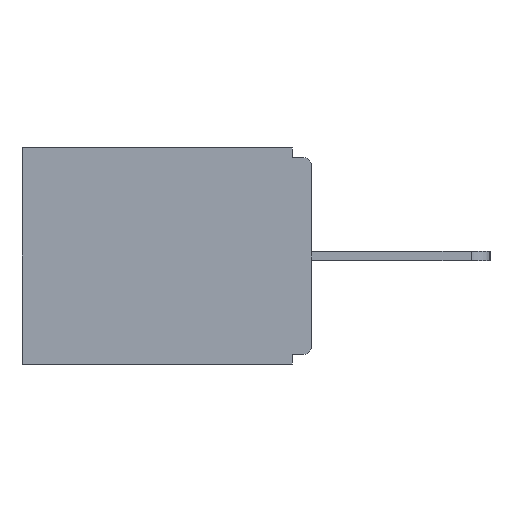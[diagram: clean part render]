
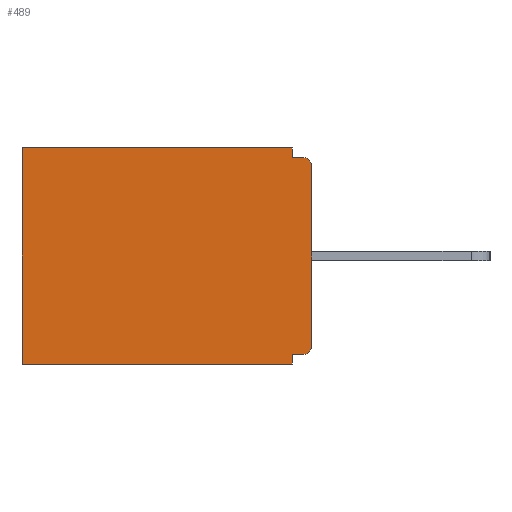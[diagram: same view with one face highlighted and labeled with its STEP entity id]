
A CAD part, left-side view. The second image highlights one B-rep face of the part: STEP entity #489.
In plain terms, the highlighted planar face has unit normal (-1, 0, 0).
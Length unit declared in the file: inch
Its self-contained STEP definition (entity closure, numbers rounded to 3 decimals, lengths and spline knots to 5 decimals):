
#12 = DIRECTION ( 'NONE',  ( 0., 0., -1. ) ) ;
#49 = ORIENTED_EDGE ( 'NONE', *, *, #7916, .T. ) ;
#286 = VECTOR ( 'NONE', #7599, 39.37008 ) ;
#290 = EDGE_CURVE ( 'NONE', #2444, #10010, #12416, .T. ) ;
#346 = CIRCLE ( 'NONE', #12971, 0.015 ) ;
#489 = ADVANCED_FACE ( 'NONE', ( #7421 ), #2189, .F. ) ;
#512 = LINE ( 'NONE', #12694, #10845 ) ;
#618 = DIRECTION ( 'NONE',  ( 0., -1., 0. ) ) ;
#804 = DIRECTION ( 'NONE',  ( 0., 0., -1. ) ) ;
#906 = ORIENTED_EDGE ( 'NONE', *, *, #11463, .F. ) ;
#972 = CARTESIAN_POINT ( 'NONE',  ( 0.298, 0.015, -0.313 ) ) ;
#1061 = CARTESIAN_POINT ( 'NONE',  ( 0.298, 0.015, -0.03 ) ) ;
#1147 = DIRECTION ( 'NONE',  ( -1., 0., 0. ) ) ;
#1415 = DIRECTION ( 'NONE',  ( 0., 1., 0. ) ) ;
#1557 = ORIENTED_EDGE ( 'NONE', *, *, #7293, .F. ) ;
#1739 = LINE ( 'NONE', #12682, #286 ) ;
#1891 = VERTEX_POINT ( 'NONE', #12522 ) ;
#1892 = DIRECTION ( 'NONE',  ( 0., 1., 0. ) ) ;
#1963 = ORIENTED_EDGE ( 'NONE', *, *, #5294, .T. ) ;
#2013 = LINE ( 'NONE', #12012, #6350 ) ;
#2139 = EDGE_LOOP ( 'NONE', ( #1963, #11850, #2563, #49, #9043, #9344, #906, #1557, #4140, #12208 ) ) ;
#2189 = PLANE ( 'NONE',  #11971 ) ;
#2194 = CARTESIAN_POINT ( 'NONE',  ( 0.298, 0.015, -0.015 ) ) ;
#2214 = CARTESIAN_POINT ( 'NONE',  ( 0.298, 0.031, -0.015 ) ) ;
#2283 = VECTOR ( 'NONE', #618, 39.37008 ) ;
#2444 = VERTEX_POINT ( 'NONE', #2214 ) ;
#2563 = ORIENTED_EDGE ( 'NONE', *, *, #6352, .F. ) ;
#2890 = CARTESIAN_POINT ( 'NONE',  ( 0.298, 0., -0.343 ) ) ;
#2955 = CARTESIAN_POINT ( 'NONE',  ( 0.298, 0., -0.03 ) ) ;
#2999 = CARTESIAN_POINT ( 'NONE',  ( 0.298, 0., 0. ) ) ;
#3053 = CARTESIAN_POINT ( 'NONE',  ( 0.298, 0.031, -0.328 ) ) ;
#3123 = LINE ( 'NONE', #12525, #12603 ) ;
#3130 = DIRECTION ( 'NONE',  ( 1., 0., 0. ) ) ;
#3139 = DIRECTION ( 'NONE',  ( 0., 0., -1. ) ) ;
#3141 = VECTOR ( 'NONE', #4086, 39.37008 ) ;
#3318 = EDGE_CURVE ( 'NONE', #7653, #8867, #8622, .T. ) ;
#4086 = DIRECTION ( 'NONE',  ( 0., 0., -1. ) ) ;
#4140 = ORIENTED_EDGE ( 'NONE', *, *, #5238, .T. ) ;
#4240 = CARTESIAN_POINT ( 'NONE',  ( 0.298, 0., 0. ) ) ;
#4428 = AXIS2_PLACEMENT_3D ( 'NONE', #972, #1147, #3139 ) ;
#5163 = DIRECTION ( 'NONE',  ( 0., 0., -1. ) ) ;
#5238 = EDGE_CURVE ( 'NONE', #5917, #8867, #8730, .T. ) ;
#5294 = EDGE_CURVE ( 'NONE', #7653, #10010, #346, .T. ) ;
#5343 = VERTEX_POINT ( 'NONE', #7398 ) ;
#5917 = VERTEX_POINT ( 'NONE', #8154 ) ;
#6086 = VERTEX_POINT ( 'NONE', #7644 ) ;
#6161 = EDGE_CURVE ( 'NONE', #1891, #5343, #11359, .T. ) ;
#6350 = VECTOR ( 'NONE', #804, 39.37008 ) ;
#6352 = EDGE_CURVE ( 'NONE', #6086, #2444, #3123, .T. ) ;
#6745 = CARTESIAN_POINT ( 'NONE',  ( 0.298, 0., -0.015 ) ) ;
#7293 = EDGE_CURVE ( 'NONE', #5917, #12135, #512, .T. ) ;
#7398 = CARTESIAN_POINT ( 'NONE',  ( 0.298, 0.46, -0.343 ) ) ;
#7421 = FACE_OUTER_BOUND ( 'NONE', #2139, .T. ) ;
#7599 = DIRECTION ( 'NONE',  ( 0., 0., -1. ) ) ;
#7644 = CARTESIAN_POINT ( 'NONE',  ( 0.298, 0.031, 0. ) ) ;
#7653 = VERTEX_POINT ( 'NONE', #2955 ) ;
#7916 = EDGE_CURVE ( 'NONE', #6086, #9658, #10833, .T. ) ;
#8071 = VECTOR ( 'NONE', #11411, 39.37008 ) ;
#8154 = CARTESIAN_POINT ( 'NONE',  ( 0.298, 0.015, -0.328 ) ) ;
#8622 = LINE ( 'NONE', #2999, #3141 ) ;
#8730 = CIRCLE ( 'NONE', #4428, 0.015 ) ;
#8867 = VERTEX_POINT ( 'NONE', #12286 ) ;
#9043 = ORIENTED_EDGE ( 'NONE', *, *, #9278, .T. ) ;
#9278 = EDGE_CURVE ( 'NONE', #9658, #5343, #1739, .T. ) ;
#9344 = ORIENTED_EDGE ( 'NONE', *, *, #6161, .F. ) ;
#9658 = VERTEX_POINT ( 'NONE', #11991 ) ;
#10010 = VERTEX_POINT ( 'NONE', #2194 ) ;
#10082 = VECTOR ( 'NONE', #1892, 39.37008 ) ;
#10272 = CARTESIAN_POINT ( 'NONE',  ( 0.298, 0., 0. ) ) ;
#10833 = LINE ( 'NONE', #4240, #8071 ) ;
#10845 = VECTOR ( 'NONE', #1415, 39.37008 ) ;
#11352 = DIRECTION ( 'NONE',  ( -1., 0., 0. ) ) ;
#11359 = LINE ( 'NONE', #2890, #10082 ) ;
#11411 = DIRECTION ( 'NONE',  ( 0., 1., 0. ) ) ;
#11463 = EDGE_CURVE ( 'NONE', #12135, #1891, #2013, .T. ) ;
#11850 = ORIENTED_EDGE ( 'NONE', *, *, #290, .F. ) ;
#11971 = AXIS2_PLACEMENT_3D ( 'NONE', #10272, #3130, #12 ) ;
#11991 = CARTESIAN_POINT ( 'NONE',  ( 0.298, 0.46, 0. ) ) ;
#12012 = CARTESIAN_POINT ( 'NONE',  ( 0.298, 0.031, -0.343 ) ) ;
#12135 = VERTEX_POINT ( 'NONE', #3053 ) ;
#12208 = ORIENTED_EDGE ( 'NONE', *, *, #3318, .F. ) ;
#12286 = CARTESIAN_POINT ( 'NONE',  ( 0.298, 0., -0.313 ) ) ;
#12416 = LINE ( 'NONE', #6745, #2283 ) ;
#12446 = DIRECTION ( 'NONE',  ( 0., 0., -1. ) ) ;
#12522 = CARTESIAN_POINT ( 'NONE',  ( 0.298, 0.031, -0.343 ) ) ;
#12525 = CARTESIAN_POINT ( 'NONE',  ( 0.298, 0.031, -0.343 ) ) ;
#12603 = VECTOR ( 'NONE', #12446, 39.37008 ) ;
#12682 = CARTESIAN_POINT ( 'NONE',  ( 0.298, 0.46, 0. ) ) ;
#12694 = CARTESIAN_POINT ( 'NONE',  ( 0.298, 0., -0.328 ) ) ;
#12971 = AXIS2_PLACEMENT_3D ( 'NONE', #1061, #11352, #5163 ) ;
